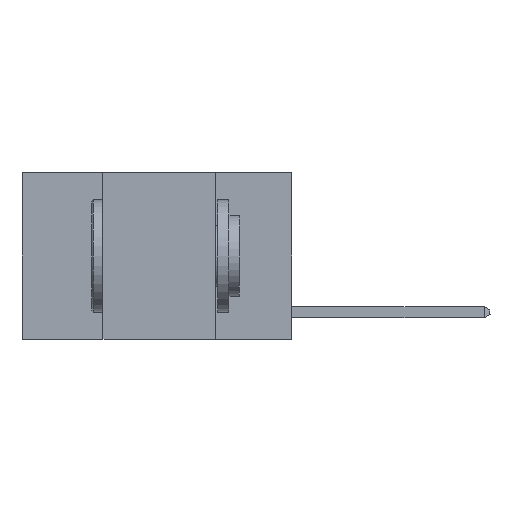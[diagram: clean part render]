
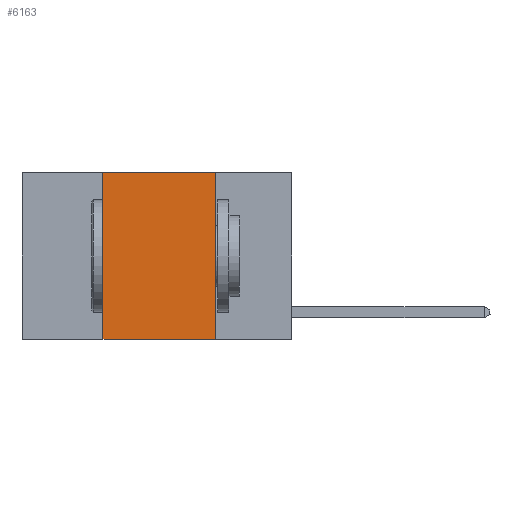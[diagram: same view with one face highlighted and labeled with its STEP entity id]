
A CAD part, left-side view. The second image highlights one B-rep face of the part: STEP entity #6163.
In plain terms, the highlighted planar face has unit normal (-1, 0, 0).
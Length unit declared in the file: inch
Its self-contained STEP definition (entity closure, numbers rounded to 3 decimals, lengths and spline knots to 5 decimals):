
#532 = VECTOR ( 'NONE', #29862, 39.37008 ) ;
#614 = CARTESIAN_POINT ( 'NONE',  ( 0., 0.17, -0.37 ) ) ;
#831 = EDGE_LOOP ( 'NONE', ( #9710, #28960, #27033, #7028 ) ) ;
#1171 = EDGE_CURVE ( 'NONE', #13200, #21401, #5079, .T. ) ;
#1997 = DIRECTION ( 'NONE',  ( 0., -1., 0. ) ) ;
#3580 = VERTEX_POINT ( 'NONE', #18433 ) ;
#3940 = CARTESIAN_POINT ( 'NONE',  ( 0., 0.42, 0. ) ) ;
#5001 = CARTESIAN_POINT ( 'NONE',  ( 0., 0.6, 0. ) ) ;
#5079 = LINE ( 'NONE', #29343, #532 ) ;
#5410 = EDGE_CURVE ( 'NONE', #21401, #3580, #21336, .T. ) ;
#6163 = ADVANCED_FACE ( 'NONE', ( #29602 ), #16690, .F. ) ;
#7028 = ORIENTED_EDGE ( 'NONE', *, *, #7671, .T. ) ;
#7671 = EDGE_CURVE ( 'NONE', #13200, #29061, #29513, .T. ) ;
#9710 = ORIENTED_EDGE ( 'NONE', *, *, #15057, .F. ) ;
#10175 = VECTOR ( 'NONE', #12470, 39.37008 ) ;
#10496 = VECTOR ( 'NONE', #14067, 39.37008 ) ;
#12470 = DIRECTION ( 'NONE',  ( 0., -1., 0. ) ) ;
#13200 = VERTEX_POINT ( 'NONE', #27352 ) ;
#13878 = CARTESIAN_POINT ( 'NONE',  ( 0., 0.17, 0. ) ) ;
#14067 = DIRECTION ( 'NONE',  ( 0., 0., -1. ) ) ;
#15057 = EDGE_CURVE ( 'NONE', #3580, #29061, #22038, .T. ) ;
#16690 = PLANE ( 'NONE',  #22906 ) ;
#16967 = VECTOR ( 'NONE', #1997, 39.37008 ) ;
#18380 = CARTESIAN_POINT ( 'NONE',  ( 0., 0.6, -0.37 ) ) ;
#18433 = CARTESIAN_POINT ( 'NONE',  ( 0., 0.17, 0. ) ) ;
#18906 = DIRECTION ( 'NONE',  ( 1., 0., 0. ) ) ;
#21281 = DIRECTION ( 'NONE',  ( 0., 0., -1. ) ) ;
#21336 = LINE ( 'NONE', #5001, #10175 ) ;
#21401 = VERTEX_POINT ( 'NONE', #3940 ) ;
#22038 = LINE ( 'NONE', #13878, #10496 ) ;
#22906 = AXIS2_PLACEMENT_3D ( 'NONE', #30654, #18906, #21281 ) ;
#27033 = ORIENTED_EDGE ( 'NONE', *, *, #1171, .F. ) ;
#27352 = CARTESIAN_POINT ( 'NONE',  ( 0., 0.42, -0.37 ) ) ;
#28960 = ORIENTED_EDGE ( 'NONE', *, *, #5410, .F. ) ;
#29061 = VERTEX_POINT ( 'NONE', #614 ) ;
#29343 = CARTESIAN_POINT ( 'NONE',  ( 0., 0.42, 0. ) ) ;
#29513 = LINE ( 'NONE', #18380, #16967 ) ;
#29602 = FACE_OUTER_BOUND ( 'NONE', #831, .T. ) ;
#29862 = DIRECTION ( 'NONE',  ( 0., 0., 1. ) ) ;
#30654 = CARTESIAN_POINT ( 'NONE',  ( 0., 0.6, 0. ) ) ;
